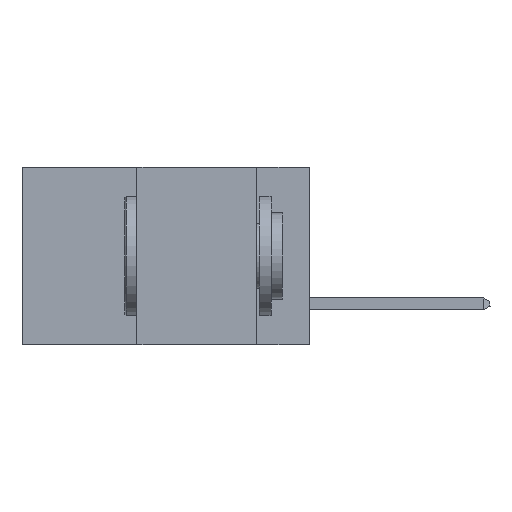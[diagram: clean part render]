
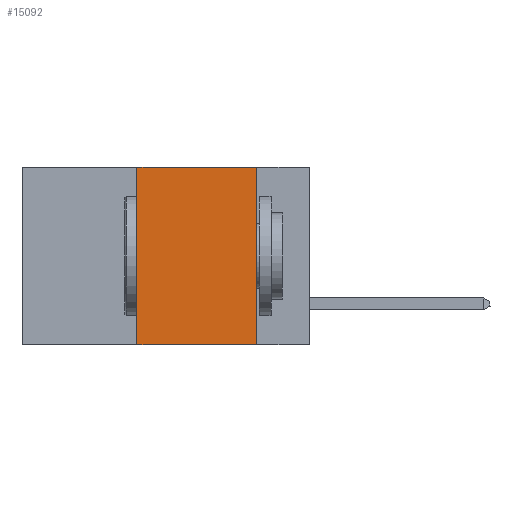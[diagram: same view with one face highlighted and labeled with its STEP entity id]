
A CAD part, left-side view. The second image highlights one B-rep face of the part: STEP entity #15092.
In plain terms, the highlighted planar face has unit normal (-1, 0, 0).
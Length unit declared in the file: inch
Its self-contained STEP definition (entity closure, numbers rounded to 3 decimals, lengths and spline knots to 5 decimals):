
#1369 = CARTESIAN_POINT ( 'NONE',  ( 0., 0.36, -0.37 ) ) ;
#1419 = CARTESIAN_POINT ( 'NONE',  ( 0., 0.6, -0.37 ) ) ;
#1580 = DIRECTION ( 'NONE',  ( 0., -1., 0. ) ) ;
#2595 = EDGE_CURVE ( 'NONE', #6066, #26126, #3875, .T. ) ;
#3875 = LINE ( 'NONE', #1419, #42460 ) ;
#4376 = ORIENTED_EDGE ( 'NONE', *, *, #19094, .F. ) ;
#5758 = LINE ( 'NONE', #12561, #14608 ) ;
#5877 = DIRECTION ( 'NONE',  ( 0., 0., -1. ) ) ;
#6066 = VERTEX_POINT ( 'NONE', #1369 ) ;
#6398 = LINE ( 'NONE', #28563, #25177 ) ;
#7615 = EDGE_CURVE ( 'NONE', #9344, #26126, #5758, .T. ) ;
#7802 = CARTESIAN_POINT ( 'NONE',  ( 0., 0.11, 0. ) ) ;
#8794 = ORIENTED_EDGE ( 'NONE', *, *, #7615, .F. ) ;
#9344 = VERTEX_POINT ( 'NONE', #7802 ) ;
#11122 = EDGE_CURVE ( 'NONE', #6066, #31656, #15971, .T. ) ;
#12561 = CARTESIAN_POINT ( 'NONE',  ( 0., 0.11, 0. ) ) ;
#14608 = VECTOR ( 'NONE', #16293, 39.37008 ) ;
#14740 = CARTESIAN_POINT ( 'NONE',  ( 0., 0.11, -0.37 ) ) ;
#15092 = ADVANCED_FACE ( 'NONE', ( #38363 ), #39405, .F. ) ;
#15971 = LINE ( 'NONE', #19200, #42228 ) ;
#16293 = DIRECTION ( 'NONE',  ( 0., 0., -1. ) ) ;
#17050 = DIRECTION ( 'NONE',  ( 1., 0., 0. ) ) ;
#17429 = DIRECTION ( 'NONE',  ( 0., -1., 0. ) ) ;
#19094 = EDGE_CURVE ( 'NONE', #31656, #9344, #6398, .T. ) ;
#19200 = CARTESIAN_POINT ( 'NONE',  ( 0., 0.36, 0. ) ) ;
#22579 = ORIENTED_EDGE ( 'NONE', *, *, #2595, .T. ) ;
#25177 = VECTOR ( 'NONE', #17429, 39.37008 ) ;
#26126 = VERTEX_POINT ( 'NONE', #14740 ) ;
#27069 = AXIS2_PLACEMENT_3D ( 'NONE', #35662, #17050, #5877 ) ;
#28563 = CARTESIAN_POINT ( 'NONE',  ( 0., 0.6, 0. ) ) ;
#30479 = DIRECTION ( 'NONE',  ( 0., 0., 1. ) ) ;
#31656 = VERTEX_POINT ( 'NONE', #43303 ) ;
#32141 = EDGE_LOOP ( 'NONE', ( #8794, #4376, #37397, #22579 ) ) ;
#35662 = CARTESIAN_POINT ( 'NONE',  ( 0., 0.6, 0. ) ) ;
#37397 = ORIENTED_EDGE ( 'NONE', *, *, #11122, .F. ) ;
#38363 = FACE_OUTER_BOUND ( 'NONE', #32141, .T. ) ;
#39405 = PLANE ( 'NONE',  #27069 ) ;
#42228 = VECTOR ( 'NONE', #30479, 39.37008 ) ;
#42460 = VECTOR ( 'NONE', #1580, 39.37008 ) ;
#43303 = CARTESIAN_POINT ( 'NONE',  ( 0., 0.36, 0. ) ) ;
